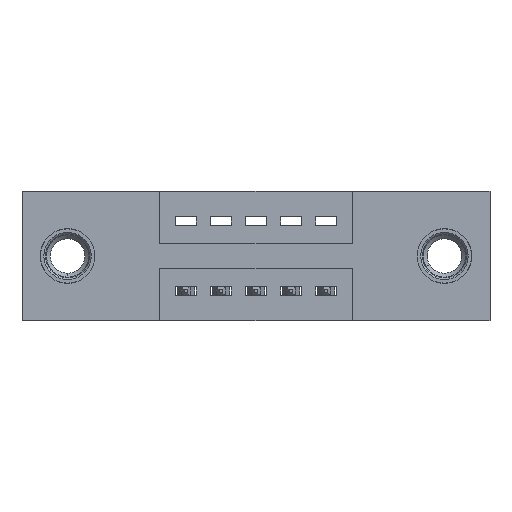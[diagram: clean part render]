
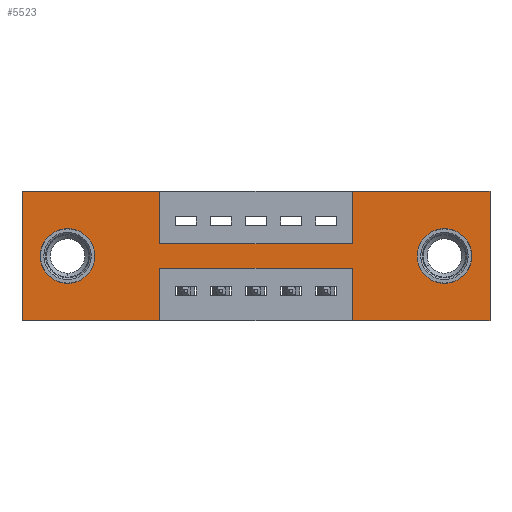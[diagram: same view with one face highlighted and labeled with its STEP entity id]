
A CAD part, front view. The second image highlights one B-rep face of the part: STEP entity #5523.
In plain terms, the highlighted planar face has unit normal (0, -1, 0).
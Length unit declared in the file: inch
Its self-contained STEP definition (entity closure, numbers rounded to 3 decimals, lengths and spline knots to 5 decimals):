
#6 = VECTOR ( 'NONE', #5009, 39.37008 ) ;
#41 = VECTOR ( 'NONE', #9210, 39.37008 ) ;
#69 = EDGE_CURVE ( 'NONE', #4238, #6413, #1591, .T. ) ;
#94 = LINE ( 'NONE', #2278, #6928 ) ;
#123 = AXIS2_PLACEMENT_3D ( 'NONE', #5217, #622, #7534 ) ;
#301 = VERTEX_POINT ( 'NONE', #8449 ) ;
#414 = EDGE_CURVE ( 'NONE', #808, #6581, #6755, .T. ) ;
#449 = VECTOR ( 'NONE', #9964, 39.37008 ) ;
#605 = DIRECTION ( 'NONE',  ( 0., 0., -1. ) ) ;
#622 = DIRECTION ( 'NONE',  ( 0., -1., 0. ) ) ;
#735 = EDGE_CURVE ( 'NONE', #5226, #5721, #4413, .T. ) ;
#777 = EDGE_LOOP ( 'NONE', ( #5458, #4737, #9768, #6508, #1508, #6535, #6142, #2093, #5713, #8961, #4875, #1519 ) ) ;
#808 = VERTEX_POINT ( 'NONE', #6233 ) ;
#945 = ORIENTED_EDGE ( 'NONE', *, *, #69, .T. ) ;
#1041 = CARTESIAN_POINT ( 'NONE',  ( 0.9425, 0., -0.15 ) ) ;
#1065 = VERTEX_POINT ( 'NONE', #9584 ) ;
#1121 = EDGE_LOOP ( 'NONE', ( #2556, #8960 ) ) ;
#1224 = CARTESIAN_POINT ( 'NONE',  ( 0.3925, 0., -0.15 ) ) ;
#1266 = VECTOR ( 'NONE', #4975, 39.37008 ) ;
#1295 = DIRECTION ( 'NONE',  ( 0., 0., 1. ) ) ;
#1508 = ORIENTED_EDGE ( 'NONE', *, *, #414, .F. ) ;
#1519 = ORIENTED_EDGE ( 'NONE', *, *, #3664, .F. ) ;
#1591 = CIRCLE ( 'NONE', #4829, 0.078 ) ;
#1680 = CARTESIAN_POINT ( 'NONE',  ( 0.13, 0., -0.263 ) ) ;
#1749 = FACE_BOUND ( 'NONE', #7635, .T. ) ;
#2058 = EDGE_CURVE ( 'NONE', #4074, #3180, #2128, .T. ) ;
#2093 = ORIENTED_EDGE ( 'NONE', *, *, #8187, .F. ) ;
#2120 = DIRECTION ( 'NONE',  ( 0., 1., 0. ) ) ;
#2128 = CIRCLE ( 'NONE', #2640, 0.078 ) ;
#2129 = DIRECTION ( 'NONE',  ( 0., 0., -1. ) ) ;
#2278 = CARTESIAN_POINT ( 'NONE',  ( 0., 0., -0.37 ) ) ;
#2401 = CARTESIAN_POINT ( 'NONE',  ( 1.335, 0., 0. ) ) ;
#2475 = AXIS2_PLACEMENT_3D ( 'NONE', #8173, #2866, #605 ) ;
#2526 = CARTESIAN_POINT ( 'NONE',  ( 0.13, 0., -0.107 ) ) ;
#2542 = DIRECTION ( 'NONE',  ( -1., 0., 0. ) ) ;
#2556 = ORIENTED_EDGE ( 'NONE', *, *, #4588, .T. ) ;
#2560 = EDGE_CURVE ( 'NONE', #6413, #4238, #5019, .T. ) ;
#2577 = CARTESIAN_POINT ( 'NONE',  ( 0., 0., -0.37 ) ) ;
#2640 = AXIS2_PLACEMENT_3D ( 'NONE', #4474, #2120, #7540 ) ;
#2694 = DIRECTION ( 'NONE',  ( -1., 0., 0. ) ) ;
#2697 = FACE_OUTER_BOUND ( 'NONE', #777, .T. ) ;
#2802 = CARTESIAN_POINT ( 'NONE',  ( 0.3925, 0., 0. ) ) ;
#2866 = DIRECTION ( 'NONE',  ( 0., 1., 0. ) ) ;
#2868 = LINE ( 'NONE', #7807, #5168 ) ;
#2895 = EDGE_CURVE ( 'NONE', #6408, #301, #8246, .T. ) ;
#2908 = CARTESIAN_POINT ( 'NONE',  ( 0.9425, 0., 0. ) ) ;
#3043 = VECTOR ( 'NONE', #2129, 39.37008 ) ;
#3080 = VERTEX_POINT ( 'NONE', #6257 ) ;
#3180 = VERTEX_POINT ( 'NONE', #4968 ) ;
#3214 = CARTESIAN_POINT ( 'NONE',  ( 0.13, 0., -0.185 ) ) ;
#3433 = CARTESIAN_POINT ( 'NONE',  ( 0., 0., 0. ) ) ;
#3493 = CARTESIAN_POINT ( 'NONE',  ( 0.9425, 0., -0.22 ) ) ;
#3531 = VECTOR ( 'NONE', #5891, 39.37008 ) ;
#3654 = VECTOR ( 'NONE', #2542, 39.37008 ) ;
#3664 = EDGE_CURVE ( 'NONE', #1065, #5851, #7728, .T. ) ;
#3823 = VERTEX_POINT ( 'NONE', #1224 ) ;
#3844 = DIRECTION ( 'NONE',  ( 0., 0., 1. ) ) ;
#4003 = VECTOR ( 'NONE', #9003, 39.37008 ) ;
#4074 = VERTEX_POINT ( 'NONE', #6000 ) ;
#4094 = LINE ( 'NONE', #5642, #4826 ) ;
#4238 = VERTEX_POINT ( 'NONE', #1680 ) ;
#4413 = LINE ( 'NONE', #2908, #4908 ) ;
#4421 = CARTESIAN_POINT ( 'NONE',  ( 0., 0., 0. ) ) ;
#4442 = PLANE ( 'NONE',  #123 ) ;
#4474 = CARTESIAN_POINT ( 'NONE',  ( 1.205, 0., -0.185 ) ) ;
#4588 = EDGE_CURVE ( 'NONE', #3180, #4074, #6197, .T. ) ;
#4708 = EDGE_CURVE ( 'NONE', #6581, #3080, #94, .T. ) ;
#4737 = ORIENTED_EDGE ( 'NONE', *, *, #2895, .F. ) ;
#4811 = LINE ( 'NONE', #7285, #6 ) ;
#4826 = VECTOR ( 'NONE', #6284, 39.37008 ) ;
#4829 = AXIS2_PLACEMENT_3D ( 'NONE', #3214, #8538, #6669 ) ;
#4875 = ORIENTED_EDGE ( 'NONE', *, *, #5919, .F. ) ;
#4908 = VECTOR ( 'NONE', #9146, 39.37008 ) ;
#4968 = CARTESIAN_POINT ( 'NONE',  ( 1.205, 0., -0.107 ) ) ;
#4975 = DIRECTION ( 'NONE',  ( 0., 0., 1. ) ) ;
#5009 = DIRECTION ( 'NONE',  ( 0., 0., -1. ) ) ;
#5019 = CIRCLE ( 'NONE', #5043, 0.078 ) ;
#5043 = AXIS2_PLACEMENT_3D ( 'NONE', #7386, #9694, #1295 ) ;
#5168 = VECTOR ( 'NONE', #3844, 39.37008 ) ;
#5191 = CARTESIAN_POINT ( 'NONE',  ( 0.3925, 0., -0.37 ) ) ;
#5217 = CARTESIAN_POINT ( 'NONE',  ( 0., 0., -0.37 ) ) ;
#5226 = VERTEX_POINT ( 'NONE', #1041 ) ;
#5439 = CARTESIAN_POINT ( 'NONE',  ( 0.3925, 0., -0.22 ) ) ;
#5458 = ORIENTED_EDGE ( 'NONE', *, *, #6558, .F. ) ;
#5523 = ADVANCED_FACE ( 'NONE', ( #8603, #1749, #2697 ), #4442, .T. ) ;
#5572 = LINE ( 'NONE', #4421, #3531 ) ;
#5642 = CARTESIAN_POINT ( 'NONE',  ( 0.3925, 0., -0.15 ) ) ;
#5708 = ORIENTED_EDGE ( 'NONE', *, *, #2560, .T. ) ;
#5713 = ORIENTED_EDGE ( 'NONE', *, *, #8815, .F. ) ;
#5721 = VERTEX_POINT ( 'NONE', #7013 ) ;
#5851 = VERTEX_POINT ( 'NONE', #8877 ) ;
#5891 = DIRECTION ( 'NONE',  ( 1., 0., 0. ) ) ;
#5919 = EDGE_CURVE ( 'NONE', #5851, #9549, #9314, .T. ) ;
#6000 = CARTESIAN_POINT ( 'NONE',  ( 1.205, 0., -0.263 ) ) ;
#6142 = ORIENTED_EDGE ( 'NONE', *, *, #735, .F. ) ;
#6197 = CIRCLE ( 'NONE', #2475, 0.078 ) ;
#6233 = CARTESIAN_POINT ( 'NONE',  ( 1.335, 0., 0. ) ) ;
#6257 = CARTESIAN_POINT ( 'NONE',  ( 0.9425, 0., -0.37 ) ) ;
#6271 = LINE ( 'NONE', #5191, #4003 ) ;
#6284 = DIRECTION ( 'NONE',  ( 1., 0., 0. ) ) ;
#6408 = VERTEX_POINT ( 'NONE', #3493 ) ;
#6413 = VERTEX_POINT ( 'NONE', #2526 ) ;
#6501 = EDGE_CURVE ( 'NONE', #5721, #808, #5572, .T. ) ;
#6508 = ORIENTED_EDGE ( 'NONE', *, *, #4708, .F. ) ;
#6535 = ORIENTED_EDGE ( 'NONE', *, *, #6501, .F. ) ;
#6558 = EDGE_CURVE ( 'NONE', #301, #1065, #6271, .T. ) ;
#6581 = VERTEX_POINT ( 'NONE', #8922 ) ;
#6669 = DIRECTION ( 'NONE',  ( 0., 0., 1. ) ) ;
#6755 = LINE ( 'NONE', #2401, #3043 ) ;
#6928 = VECTOR ( 'NONE', #2694, 39.37008 ) ;
#7013 = CARTESIAN_POINT ( 'NONE',  ( 0.9425, 0., 0. ) ) ;
#7161 = VERTEX_POINT ( 'NONE', #2802 ) ;
#7222 = EDGE_CURVE ( 'NONE', #9549, #7161, #8935, .T. ) ;
#7267 = CARTESIAN_POINT ( 'NONE',  ( 0., 0., 0. ) ) ;
#7285 = CARTESIAN_POINT ( 'NONE',  ( 0.3925, 0., 0. ) ) ;
#7386 = CARTESIAN_POINT ( 'NONE',  ( 0.13, 0., -0.185 ) ) ;
#7534 = DIRECTION ( 'NONE',  ( 0., 0., -1. ) ) ;
#7540 = DIRECTION ( 'NONE',  ( 0., 0., -1. ) ) ;
#7635 = EDGE_LOOP ( 'NONE', ( #5708, #945 ) ) ;
#7728 = LINE ( 'NONE', #2577, #3654 ) ;
#7807 = CARTESIAN_POINT ( 'NONE',  ( 0.9425, 0., -0.37 ) ) ;
#8173 = CARTESIAN_POINT ( 'NONE',  ( 1.205, 0., -0.185 ) ) ;
#8187 = EDGE_CURVE ( 'NONE', #3823, #5226, #4094, .T. ) ;
#8246 = LINE ( 'NONE', #5439, #449 ) ;
#8449 = CARTESIAN_POINT ( 'NONE',  ( 0.3925, 0., -0.22 ) ) ;
#8538 = DIRECTION ( 'NONE',  ( 0., 1., 0. ) ) ;
#8603 = FACE_BOUND ( 'NONE', #1121, .T. ) ;
#8815 = EDGE_CURVE ( 'NONE', #7161, #3823, #4811, .T. ) ;
#8877 = CARTESIAN_POINT ( 'NONE',  ( 0., 0., -0.37 ) ) ;
#8922 = CARTESIAN_POINT ( 'NONE',  ( 1.335, 0., -0.37 ) ) ;
#8935 = LINE ( 'NONE', #9071, #41 ) ;
#8960 = ORIENTED_EDGE ( 'NONE', *, *, #2058, .T. ) ;
#8961 = ORIENTED_EDGE ( 'NONE', *, *, #7222, .F. ) ;
#9003 = DIRECTION ( 'NONE',  ( 0., 0., -1. ) ) ;
#9071 = CARTESIAN_POINT ( 'NONE',  ( 0., 0., 0. ) ) ;
#9146 = DIRECTION ( 'NONE',  ( 0., 0., 1. ) ) ;
#9210 = DIRECTION ( 'NONE',  ( 1., 0., 0. ) ) ;
#9251 = EDGE_CURVE ( 'NONE', #3080, #6408, #2868, .T. ) ;
#9314 = LINE ( 'NONE', #3433, #1266 ) ;
#9549 = VERTEX_POINT ( 'NONE', #7267 ) ;
#9584 = CARTESIAN_POINT ( 'NONE',  ( 0.3925, 0., -0.37 ) ) ;
#9694 = DIRECTION ( 'NONE',  ( 0., 1., 0. ) ) ;
#9768 = ORIENTED_EDGE ( 'NONE', *, *, #9251, .F. ) ;
#9964 = DIRECTION ( 'NONE',  ( -1., 0., 0. ) ) ;
